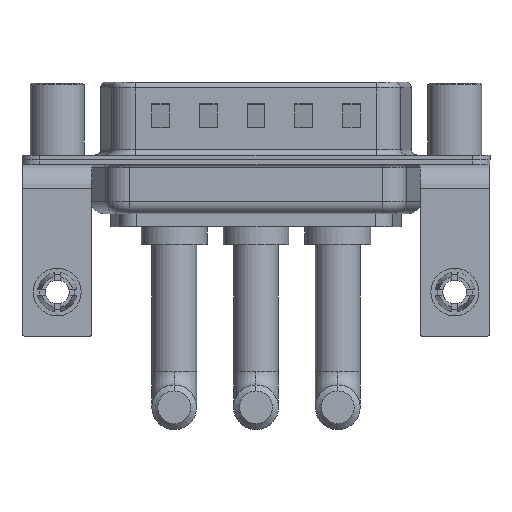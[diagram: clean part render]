
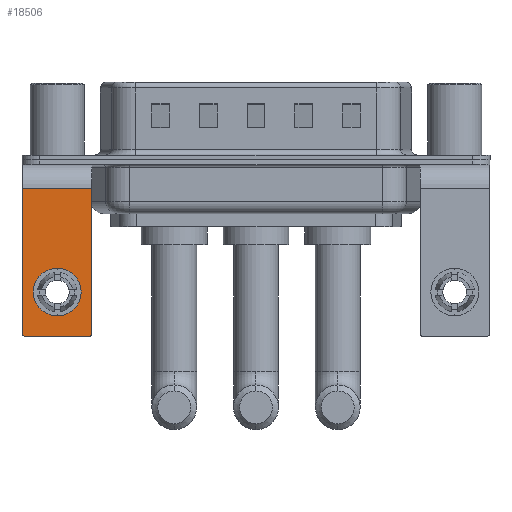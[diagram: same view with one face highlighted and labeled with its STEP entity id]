
A CAD part, front view. The second image highlights one B-rep face of the part: STEP entity #18506.
In plain terms, the highlighted planar face has unit normal (0, -1, 0).
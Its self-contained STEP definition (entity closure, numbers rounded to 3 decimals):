
#343 = DIRECTION ( 'NONE',  ( 0., 1., 0. ) ) ;
#628 = VERTEX_POINT ( 'NONE', #15716 ) ;
#828 = EDGE_CURVE ( 'NONE', #628, #8531, #5735, .T. ) ;
#1373 = CARTESIAN_POINT ( 'NONE',  ( 0., -6.25, -11.07 ) ) ;
#1797 = EDGE_CURVE ( 'NONE', #5728, #14936, #13047, .T. ) ;
#2627 = LINE ( 'NONE', #14572, #6179 ) ;
#2840 = VERTEX_POINT ( 'NONE', #5967 ) ;
#3159 = CARTESIAN_POINT ( 'NONE',  ( 2.9, -6.25, -2.4 ) ) ;
#3352 = AXIS2_PLACEMENT_3D ( 'NONE', #1373, #19811, #7489 ) ;
#3440 = CARTESIAN_POINT ( 'NONE',  ( 2.9, -6.25, -2.4 ) ) ;
#4026 = CIRCLE ( 'NONE', #11382, 2. ) ;
#4811 = CARTESIAN_POINT ( 'NONE',  ( 0., -6.25, -13.07 ) ) ;
#4919 = VERTEX_POINT ( 'NONE', #15727 ) ;
#5216 = EDGE_LOOP ( 'NONE', ( #15999, #14316, #9777, #6570, #19681, #9774 ) ) ;
#5249 = FACE_OUTER_BOUND ( 'NONE', #5216, .T. ) ;
#5728 = VERTEX_POINT ( 'NONE', #18989 ) ;
#5735 = LINE ( 'NONE', #12056, #9288 ) ;
#5867 = CARTESIAN_POINT ( 'NONE',  ( -2.9, -6.25, -14.55 ) ) ;
#5967 = CARTESIAN_POINT ( 'NONE',  ( 0., -6.25, -9.07 ) ) ;
#6179 = VECTOR ( 'NONE', #12963, 1000. ) ;
#6570 = ORIENTED_EDGE ( 'NONE', *, *, #6590, .T. ) ;
#6590 = EDGE_CURVE ( 'NONE', #628, #19169, #8247, .T. ) ;
#7030 = VECTOR ( 'NONE', #7138, 1000. ) ;
#7138 = DIRECTION ( 'NONE',  ( 0., 0., -1. ) ) ;
#7293 = AXIS2_PLACEMENT_3D ( 'NONE', #11700, #17811, #19411 ) ;
#7489 = DIRECTION ( 'NONE',  ( 0., 0., 1. ) ) ;
#8071 = DIRECTION ( 'NONE',  ( 0., 0., 1. ) ) ;
#8247 = CIRCLE ( 'NONE', #7293, 0.25 ) ;
#8531 = VERTEX_POINT ( 'NONE', #8869 ) ;
#8581 = DIRECTION ( 'NONE',  ( 0., -1., 0. ) ) ;
#8869 = CARTESIAN_POINT ( 'NONE',  ( -2.65, -6.25, -14.8 ) ) ;
#9069 = CARTESIAN_POINT ( 'NONE',  ( 2.9, -6.25, -14.55 ) ) ;
#9284 = DIRECTION ( 'NONE',  ( -1., 0., 0. ) ) ;
#9288 = VECTOR ( 'NONE', #19370, 1000. ) ;
#9774 = ORIENTED_EDGE ( 'NONE', *, *, #11153, .T. ) ;
#9777 = ORIENTED_EDGE ( 'NONE', *, *, #828, .F. ) ;
#10388 = AXIS2_PLACEMENT_3D ( 'NONE', #13203, #8581, #14705 ) ;
#10972 = DIRECTION ( 'NONE',  ( 0., 0., 1. ) ) ;
#11153 = EDGE_CURVE ( 'NONE', #4919, #5728, #16902, .T. ) ;
#11382 = AXIS2_PLACEMENT_3D ( 'NONE', #16991, #18588, #10972 ) ;
#11642 = CARTESIAN_POINT ( 'NONE',  ( -2.9, -6.25, -2.4 ) ) ;
#11700 = CARTESIAN_POINT ( 'NONE',  ( 2.65, -6.25, -14.55 ) ) ;
#11737 = EDGE_CURVE ( 'NONE', #4919, #19169, #2627, .T. ) ;
#12056 = CARTESIAN_POINT ( 'NONE',  ( 2.9, -6.25, -14.8 ) ) ;
#12963 = DIRECTION ( 'NONE',  ( 0., 0., -1. ) ) ;
#13047 = LINE ( 'NONE', #11642, #7030 ) ;
#13203 = CARTESIAN_POINT ( 'NONE',  ( -2.65, -6.25, -14.55 ) ) ;
#14191 = PLANE ( 'NONE',  #16266 ) ;
#14235 = EDGE_CURVE ( 'NONE', #16103, #2840, #18125, .T. ) ;
#14316 = ORIENTED_EDGE ( 'NONE', *, *, #18207, .T. ) ;
#14486 = ORIENTED_EDGE ( 'NONE', *, *, #14235, .T. ) ;
#14550 = EDGE_LOOP ( 'NONE', ( #14486, #19429 ) ) ;
#14572 = CARTESIAN_POINT ( 'NONE',  ( 2.9, -6.25, -2.4 ) ) ;
#14705 = DIRECTION ( 'NONE',  ( 0., 0., 1. ) ) ;
#14936 = VERTEX_POINT ( 'NONE', #5867 ) ;
#15180 = EDGE_CURVE ( 'NONE', #2840, #16103, #4026, .T. ) ;
#15716 = CARTESIAN_POINT ( 'NONE',  ( 2.65, -6.25, -14.8 ) ) ;
#15727 = CARTESIAN_POINT ( 'NONE',  ( 2.9, -6.25, -2.4 ) ) ;
#15791 = FACE_BOUND ( 'NONE', #14550, .T. ) ;
#15999 = ORIENTED_EDGE ( 'NONE', *, *, #1797, .T. ) ;
#16103 = VERTEX_POINT ( 'NONE', #4811 ) ;
#16266 = AXIS2_PLACEMENT_3D ( 'NONE', #3440, #343, #8071 ) ;
#16805 = CIRCLE ( 'NONE', #10388, 0.25 ) ;
#16902 = LINE ( 'NONE', #3159, #18642 ) ;
#16991 = CARTESIAN_POINT ( 'NONE',  ( 0., -6.25, -11.07 ) ) ;
#17811 = DIRECTION ( 'NONE',  ( 0., -1., 0. ) ) ;
#18125 = CIRCLE ( 'NONE', #3352, 2. ) ;
#18207 = EDGE_CURVE ( 'NONE', #14936, #8531, #16805, .T. ) ;
#18506 = ADVANCED_FACE ( 'NONE', ( #15791, #5249 ), #14191, .F. ) ;
#18588 = DIRECTION ( 'NONE',  ( 0., 1., 0. ) ) ;
#18642 = VECTOR ( 'NONE', #9284, 1000. ) ;
#18989 = CARTESIAN_POINT ( 'NONE',  ( -2.9, -6.25, -2.4 ) ) ;
#19169 = VERTEX_POINT ( 'NONE', #9069 ) ;
#19370 = DIRECTION ( 'NONE',  ( -1., 0., 0. ) ) ;
#19411 = DIRECTION ( 'NONE',  ( 0., 0., 1. ) ) ;
#19429 = ORIENTED_EDGE ( 'NONE', *, *, #15180, .T. ) ;
#19681 = ORIENTED_EDGE ( 'NONE', *, *, #11737, .F. ) ;
#19811 = DIRECTION ( 'NONE',  ( 0., 1., 0. ) ) ;
